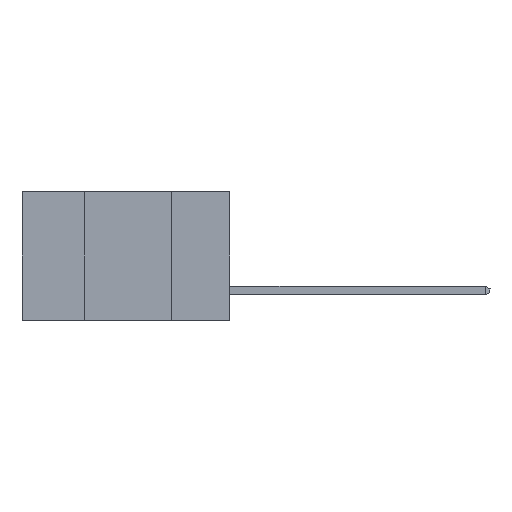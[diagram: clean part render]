
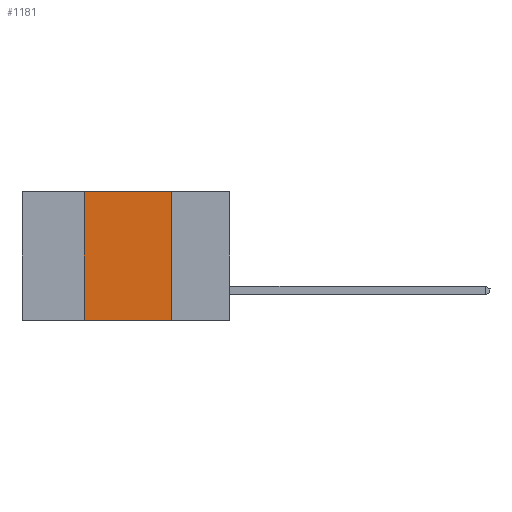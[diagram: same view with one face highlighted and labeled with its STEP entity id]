
A CAD part, left-side view. The second image highlights one B-rep face of the part: STEP entity #1181.
In plain terms, the highlighted planar face has unit normal (-1, 0, 0).
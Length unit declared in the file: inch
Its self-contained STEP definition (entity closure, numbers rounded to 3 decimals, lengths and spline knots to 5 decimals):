
#95 = EDGE_LOOP ( 'NONE', ( #22684, #6240, #11982, #13815 ) ) ;
#271 = VECTOR ( 'NONE', #18398, 39.37008 ) ;
#1181 = ADVANCED_FACE ( 'NONE', ( #1213 ), #2510, .F. ) ;
#1213 = FACE_OUTER_BOUND ( 'NONE', #95, .T. ) ;
#1333 = VERTEX_POINT ( 'NONE', #13559 ) ;
#1769 = DIRECTION ( 'NONE',  ( 0., -1., 0. ) ) ;
#2479 = DIRECTION ( 'NONE',  ( 0., 0., -1. ) ) ;
#2484 = DIRECTION ( 'NONE',  ( 1., 0., 0. ) ) ;
#2510 = PLANE ( 'NONE',  #9828 ) ;
#2799 = LINE ( 'NONE', #22624, #21705 ) ;
#3224 = CARTESIAN_POINT ( 'NONE',  ( 0., 0.6, 0. ) ) ;
#3252 = EDGE_CURVE ( 'NONE', #6047, #13701, #14785, .T. ) ;
#4578 = CARTESIAN_POINT ( 'NONE',  ( 0., 0.17, -0.37 ) ) ;
#5168 = CARTESIAN_POINT ( 'NONE',  ( 0., 0.6, -0.37 ) ) ;
#5395 = LINE ( 'NONE', #5168, #271 ) ;
#5850 = EDGE_CURVE ( 'NONE', #1333, #7505, #11162, .T. ) ;
#6047 = VERTEX_POINT ( 'NONE', #17358 ) ;
#6240 = ORIENTED_EDGE ( 'NONE', *, *, #11783, .F. ) ;
#7505 = VERTEX_POINT ( 'NONE', #4578 ) ;
#9828 = AXIS2_PLACEMENT_3D ( 'NONE', #3224, #2484, #2479 ) ;
#11162 = LINE ( 'NONE', #24194, #20488 ) ;
#11446 = CARTESIAN_POINT ( 'NONE',  ( 0., 0.42, 0. ) ) ;
#11783 = EDGE_CURVE ( 'NONE', #13701, #1333, #2799, .T. ) ;
#11982 = ORIENTED_EDGE ( 'NONE', *, *, #3252, .F. ) ;
#13132 = DIRECTION ( 'NONE',  ( 0., 0., -1. ) ) ;
#13559 = CARTESIAN_POINT ( 'NONE',  ( 0., 0.17, 0. ) ) ;
#13652 = CARTESIAN_POINT ( 'NONE',  ( 0., 0.42, -0.37 ) ) ;
#13701 = VERTEX_POINT ( 'NONE', #11446 ) ;
#13815 = ORIENTED_EDGE ( 'NONE', *, *, #15709, .T. ) ;
#14219 = DIRECTION ( 'NONE',  ( 0., 0., 1. ) ) ;
#14785 = LINE ( 'NONE', #13652, #19120 ) ;
#15709 = EDGE_CURVE ( 'NONE', #6047, #7505, #5395, .T. ) ;
#17358 = CARTESIAN_POINT ( 'NONE',  ( 0., 0.42, -0.37 ) ) ;
#18398 = DIRECTION ( 'NONE',  ( 0., -1., 0. ) ) ;
#19120 = VECTOR ( 'NONE', #14219, 39.37008 ) ;
#20488 = VECTOR ( 'NONE', #13132, 39.37008 ) ;
#21705 = VECTOR ( 'NONE', #1769, 39.37008 ) ;
#22624 = CARTESIAN_POINT ( 'NONE',  ( 0., 0.6, 0. ) ) ;
#22684 = ORIENTED_EDGE ( 'NONE', *, *, #5850, .F. ) ;
#24194 = CARTESIAN_POINT ( 'NONE',  ( 0., 0.17, -0.37 ) ) ;
